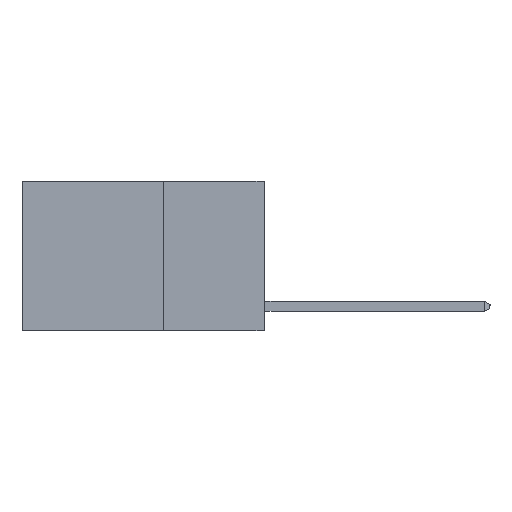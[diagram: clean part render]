
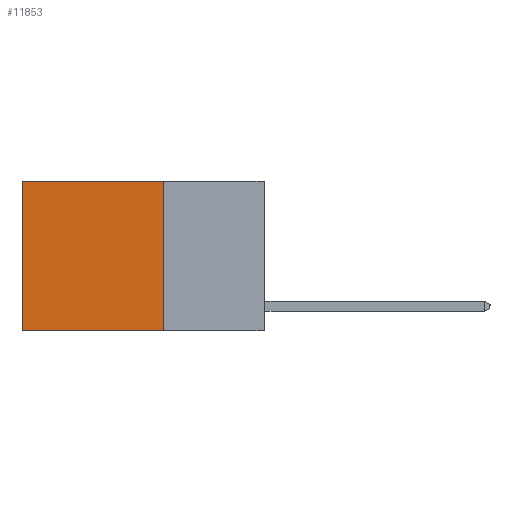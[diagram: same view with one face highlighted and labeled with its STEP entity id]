
A CAD part, left-side view. The second image highlights one B-rep face of the part: STEP entity #11853.
In plain terms, the highlighted planar face has unit normal (-1, 0, 0).
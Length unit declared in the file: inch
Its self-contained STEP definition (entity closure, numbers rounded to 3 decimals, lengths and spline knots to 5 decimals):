
#495 = CARTESIAN_POINT ( 'NONE',  ( 0.2625, 0.25, 0. ) ) ;
#665 = VECTOR ( 'NONE', #6609, 39.37008 ) ;
#762 = ORIENTED_EDGE ( 'NONE', *, *, #3541, .F. ) ;
#1114 = VECTOR ( 'NONE', #8518, 39.37008 ) ;
#1145 = VERTEX_POINT ( 'NONE', #8832 ) ;
#1990 = CARTESIAN_POINT ( 'NONE',  ( 0.2625, 0.25, 0. ) ) ;
#2831 = EDGE_CURVE ( 'NONE', #13935, #1145, #11517, .T. ) ;
#2904 = FACE_OUTER_BOUND ( 'NONE', #12228, .T. ) ;
#2930 = ORIENTED_EDGE ( 'NONE', *, *, #11069, .T. ) ;
#2936 = DIRECTION ( 'NONE',  ( 0., 1., 0. ) ) ;
#3288 = DIRECTION ( 'NONE',  ( 1., 0., 0. ) ) ;
#3541 = EDGE_CURVE ( 'NONE', #11203, #13462, #8003, .T. ) ;
#4329 = VECTOR ( 'NONE', #2936, 39.37008 ) ;
#5226 = VECTOR ( 'NONE', #13323, 39.37008 ) ;
#5330 = CARTESIAN_POINT ( 'NONE',  ( 0.2625, 0.25, -0.37 ) ) ;
#5541 = CARTESIAN_POINT ( 'NONE',  ( 0.2625, 0.25, 0. ) ) ;
#6609 = DIRECTION ( 'NONE',  ( 0., 1., 0. ) ) ;
#7132 = CARTESIAN_POINT ( 'NONE',  ( 0.2625, 0.6, 0. ) ) ;
#7214 = CARTESIAN_POINT ( 'NONE',  ( 0.2625, 0.25, 0. ) ) ;
#7934 = CARTESIAN_POINT ( 'NONE',  ( 0.2625, 0.25, -0.37 ) ) ;
#8003 = LINE ( 'NONE', #7214, #1114 ) ;
#8428 = AXIS2_PLACEMENT_3D ( 'NONE', #1990, #3288, #12140 ) ;
#8518 = DIRECTION ( 'NONE',  ( 0., 0., -1. ) ) ;
#8832 = CARTESIAN_POINT ( 'NONE',  ( 0.2625, 0.6, -0.37 ) ) ;
#9683 = PLANE ( 'NONE',  #8428 ) ;
#10527 = LINE ( 'NONE', #5330, #665 ) ;
#10706 = LINE ( 'NONE', #5541, #4329 ) ;
#11069 = EDGE_CURVE ( 'NONE', #11203, #13935, #10706, .T. ) ;
#11203 = VERTEX_POINT ( 'NONE', #495 ) ;
#11329 = ORIENTED_EDGE ( 'NONE', *, *, #14004, .F. ) ;
#11517 = LINE ( 'NONE', #7132, #5226 ) ;
#11824 = ORIENTED_EDGE ( 'NONE', *, *, #2831, .T. ) ;
#11853 = ADVANCED_FACE ( 'NONE', ( #2904 ), #9683, .F. ) ;
#12140 = DIRECTION ( 'NONE',  ( 0., 0., -1. ) ) ;
#12228 = EDGE_LOOP ( 'NONE', ( #11824, #11329, #762, #2930 ) ) ;
#13323 = DIRECTION ( 'NONE',  ( 0., 0., -1. ) ) ;
#13462 = VERTEX_POINT ( 'NONE', #7934 ) ;
#13935 = VERTEX_POINT ( 'NONE', #15114 ) ;
#14004 = EDGE_CURVE ( 'NONE', #13462, #1145, #10527, .T. ) ;
#15114 = CARTESIAN_POINT ( 'NONE',  ( 0.2625, 0.6, 0. ) ) ;
